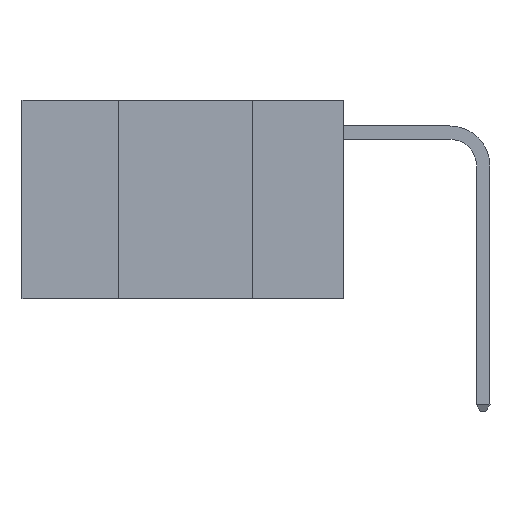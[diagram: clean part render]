
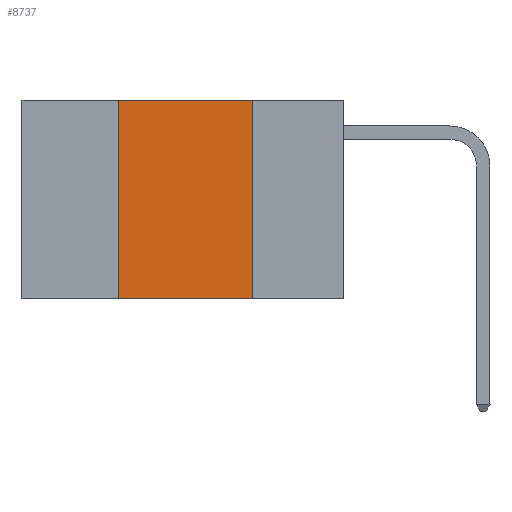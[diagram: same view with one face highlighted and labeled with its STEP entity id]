
A CAD part, left-side view. The second image highlights one B-rep face of the part: STEP entity #8737.
In plain terms, the highlighted planar face has unit normal (-1, 0, 0).
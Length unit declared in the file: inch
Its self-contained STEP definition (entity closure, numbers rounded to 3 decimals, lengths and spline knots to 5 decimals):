
#573 = VERTEX_POINT ( 'NONE', #12595 ) ;
#1137 = ORIENTED_EDGE ( 'NONE', *, *, #17450, .F. ) ;
#1214 = LINE ( 'NONE', #14653, #22016 ) ;
#1229 = LINE ( 'NONE', #4468, #10973 ) ;
#2621 = LINE ( 'NONE', #9443, #20043 ) ;
#2858 = ORIENTED_EDGE ( 'NONE', *, *, #18410, .F. ) ;
#3166 = CARTESIAN_POINT ( 'NONE',  ( 0., 0.6, 0. ) ) ;
#4468 = CARTESIAN_POINT ( 'NONE',  ( 0., 0.6, -0.37 ) ) ;
#4952 = FACE_OUTER_BOUND ( 'NONE', #17571, .T. ) ;
#5800 = ORIENTED_EDGE ( 'NONE', *, *, #16550, .F. ) ;
#6635 = CARTESIAN_POINT ( 'NONE',  ( 0., 0.42, 0. ) ) ;
#7225 = EDGE_CURVE ( 'NONE', #7293, #9795, #1229, .T. ) ;
#7293 = VERTEX_POINT ( 'NONE', #12752 ) ;
#8412 = VERTEX_POINT ( 'NONE', #17421 ) ;
#8702 = VECTOR ( 'NONE', #16771, 39.37008 ) ;
#8737 = ADVANCED_FACE ( 'NONE', ( #4952 ), #18537, .F. ) ;
#9443 = CARTESIAN_POINT ( 'NONE',  ( 0., 0.17, 0. ) ) ;
#9795 = VERTEX_POINT ( 'NONE', #10326 ) ;
#10326 = CARTESIAN_POINT ( 'NONE',  ( 0., 0.17, -0.37 ) ) ;
#10973 = VECTOR ( 'NONE', #16255, 39.37008 ) ;
#11250 = LINE ( 'NONE', #6635, #8702 ) ;
#12595 = CARTESIAN_POINT ( 'NONE',  ( 0., 0.17, 0. ) ) ;
#12752 = CARTESIAN_POINT ( 'NONE',  ( 0., 0.42, -0.37 ) ) ;
#14587 = DIRECTION ( 'NONE',  ( 0., 0., -1. ) ) ;
#14653 = CARTESIAN_POINT ( 'NONE',  ( 0., 0.6, 0. ) ) ;
#15241 = DIRECTION ( 'NONE',  ( 0., 0., -1. ) ) ;
#16255 = DIRECTION ( 'NONE',  ( 0., -1., 0. ) ) ;
#16550 = EDGE_CURVE ( 'NONE', #573, #9795, #2621, .T. ) ;
#16771 = DIRECTION ( 'NONE',  ( 0., 0., 1. ) ) ;
#16956 = DIRECTION ( 'NONE',  ( 1., 0., 0. ) ) ;
#17244 = ORIENTED_EDGE ( 'NONE', *, *, #7225, .T. ) ;
#17421 = CARTESIAN_POINT ( 'NONE',  ( 0., 0.42, 0. ) ) ;
#17450 = EDGE_CURVE ( 'NONE', #8412, #573, #1214, .T. ) ;
#17571 = EDGE_LOOP ( 'NONE', ( #5800, #1137, #2858, #17244 ) ) ;
#18282 = DIRECTION ( 'NONE',  ( 0., -1., 0. ) ) ;
#18410 = EDGE_CURVE ( 'NONE', #7293, #8412, #11250, .T. ) ;
#18537 = PLANE ( 'NONE',  #21466 ) ;
#20043 = VECTOR ( 'NONE', #14587, 39.37008 ) ;
#21466 = AXIS2_PLACEMENT_3D ( 'NONE', #3166, #16956, #15241 ) ;
#22016 = VECTOR ( 'NONE', #18282, 39.37008 ) ;
